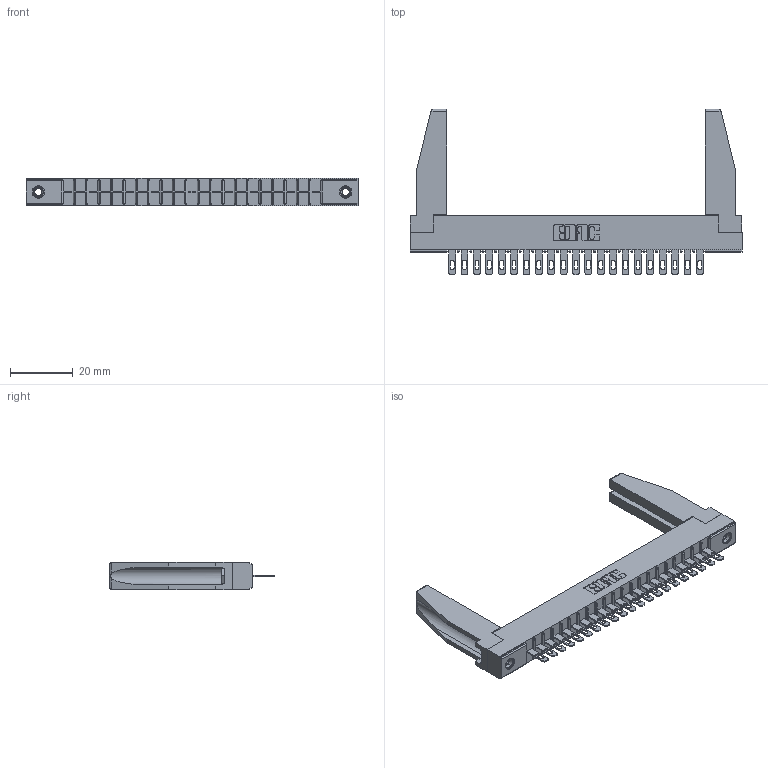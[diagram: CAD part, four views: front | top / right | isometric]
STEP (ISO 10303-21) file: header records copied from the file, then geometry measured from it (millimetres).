
FILE_DESCRIPTION (( 'STEP AP203' ), '1' );
FILE_NAME ('306-021-500-178.STEP', '2019-09-11T20:48:43', ( '' ), ( '' ), 'SwSTEP 2.0', 'SolidWorks 2016', '' );
FILE_SCHEMA (( 'CONFIG_CONTROL_DESIGN' ));
Length unit declared in the file: inch
Products named in the file (5): 345-250-001_345-250-001-102; 306-290-001_100; 306-021-500-178; 307-220-078; 306 Part_.156 Dia
Assembly tree (26 placements, depth 2):
  306-021-500-178
    306 Part_.156 Dia
    306-290-001_100  x21
    345-250-001_345-250-001-102  x2
    307-220-078  x2
Bounding box: 106.22 x 52.91 x 8.71 mm (x, y, z)
Volume: 11317.3 mm3; surface area: 14969.5 mm2
Topology: 26 solids, 26 shells, 1842 faces, 5161 edges, 3318 vertices
Faces by surface type: plane 1202, cylinder 540, sphere 84, cone 12, torus 4
Entity records: 24907 total; most frequent: CARTESIAN_POINT 4180, ORIENTED_EDGE 4100, DIRECTION 4076, EDGE_CURVE 2050, VECTOR 1592, LINE 1592, VERTEX_POINT 1304, AXIS2_PLACEMENT_3D 1242
